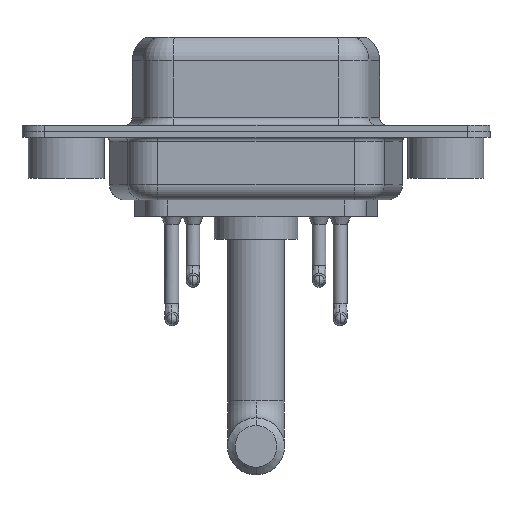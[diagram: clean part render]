
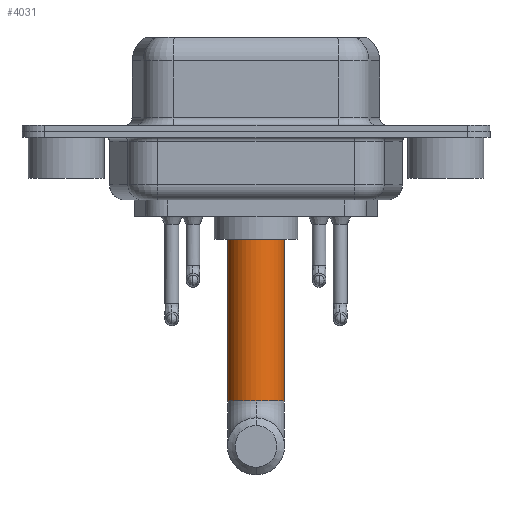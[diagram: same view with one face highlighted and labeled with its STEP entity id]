
A CAD part, front view. The second image highlights one B-rep face of the part: STEP entity #4031.
In plain terms, the highlighted cylindrical face has radius 1.875 mm (diameter 3.75 mm), a partial arc.
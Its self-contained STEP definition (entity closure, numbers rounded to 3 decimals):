
#170 = DIRECTION ( 'NONE',  ( 0., 0., -1. ) ) ;
#343 = CYLINDRICAL_SURFACE ( 'NONE', #12474, 1.875 ) ;
#483 = VERTEX_POINT ( 'NONE', #9952 ) ;
#507 = VERTEX_POINT ( 'NONE', #10357 ) ;
#1009 = ORIENTED_EDGE ( 'NONE', *, *, #11623, .F. ) ;
#1111 = DIRECTION ( 'NONE',  ( 0., 0., -1. ) ) ;
#1263 = AXIS2_PLACEMENT_3D ( 'NONE', #15798, #8086, #3154 ) ;
#1692 = ORIENTED_EDGE ( 'NONE', *, *, #10948, .T. ) ;
#1806 = DIRECTION ( 'NONE',  ( -1., 0., 0. ) ) ;
#2288 = DIRECTION ( 'NONE',  ( 0., 0., -1. ) ) ;
#2350 = CARTESIAN_POINT ( 'NONE',  ( -1.875, 0., 0. ) ) ;
#2903 = FACE_OUTER_BOUND ( 'NONE', #8813, .T. ) ;
#3154 = DIRECTION ( 'NONE',  ( -1., 0., 0. ) ) ;
#3220 = VECTOR ( 'NONE', #2288, 1000. ) ;
#3273 = DIRECTION ( 'NONE',  ( 0., 0., -1. ) ) ;
#3351 = CARTESIAN_POINT ( 'NONE',  ( 0., 0., 0. ) ) ;
#4031 = ADVANCED_FACE ( 'NONE', ( #2903 ), #343, .T. ) ;
#5236 = CARTESIAN_POINT ( 'NONE',  ( 1.875, 0., -10.63 ) ) ;
#5381 = CARTESIAN_POINT ( 'NONE',  ( 0., 0., 0. ) ) ;
#5543 = CIRCLE ( 'NONE', #15495, 1.875 ) ;
#5812 = CARTESIAN_POINT ( 'NONE',  ( 1.875, 0., 0. ) ) ;
#5974 = LINE ( 'NONE', #5812, #3220 ) ;
#6690 = EDGE_CURVE ( 'NONE', #12881, #10483, #8356, .T. ) ;
#6854 = CIRCLE ( 'NONE', #13939, 1.875 ) ;
#6868 = VERTEX_POINT ( 'NONE', #5236 ) ;
#8086 = DIRECTION ( 'NONE',  ( 0., 0., -1. ) ) ;
#8356 = LINE ( 'NONE', #2350, #13434 ) ;
#8684 = EDGE_CURVE ( 'NONE', #507, #10483, #14648, .T. ) ;
#8813 = EDGE_LOOP ( 'NONE', ( #14746, #1692, #15612, #9392, #1009 ) ) ;
#9392 = ORIENTED_EDGE ( 'NONE', *, *, #8684, .F. ) ;
#9952 = CARTESIAN_POINT ( 'NONE',  ( 1.875, 0., 0. ) ) ;
#10357 = CARTESIAN_POINT ( 'NONE',  ( 0., -1.875, -10.63 ) ) ;
#10393 = DIRECTION ( 'NONE',  ( 0., 0., -1. ) ) ;
#10483 = VERTEX_POINT ( 'NONE', #13395 ) ;
#10948 = EDGE_CURVE ( 'NONE', #483, #12881, #5543, .T. ) ;
#11623 = EDGE_CURVE ( 'NONE', #6868, #507, #6854, .T. ) ;
#12474 = AXIS2_PLACEMENT_3D ( 'NONE', #5381, #10393, #15392 ) ;
#12518 = CARTESIAN_POINT ( 'NONE',  ( 0., 0., -10.63 ) ) ;
#12767 = EDGE_CURVE ( 'NONE', #483, #6868, #5974, .T. ) ;
#12881 = VERTEX_POINT ( 'NONE', #13545 ) ;
#13395 = CARTESIAN_POINT ( 'NONE',  ( -1.875, 0., -10.63 ) ) ;
#13434 = VECTOR ( 'NONE', #1111, 1000. ) ;
#13545 = CARTESIAN_POINT ( 'NONE',  ( -1.875, 0., 0. ) ) ;
#13661 = DIRECTION ( 'NONE',  ( -1., 0., 0. ) ) ;
#13939 = AXIS2_PLACEMENT_3D ( 'NONE', #12518, #170, #13661 ) ;
#14648 = CIRCLE ( 'NONE', #1263, 1.875 ) ;
#14746 = ORIENTED_EDGE ( 'NONE', *, *, #12767, .F. ) ;
#15392 = DIRECTION ( 'NONE',  ( -1., 0., 0. ) ) ;
#15495 = AXIS2_PLACEMENT_3D ( 'NONE', #3351, #3273, #1806 ) ;
#15612 = ORIENTED_EDGE ( 'NONE', *, *, #6690, .T. ) ;
#15798 = CARTESIAN_POINT ( 'NONE',  ( 0., 0., -10.63 ) ) ;
